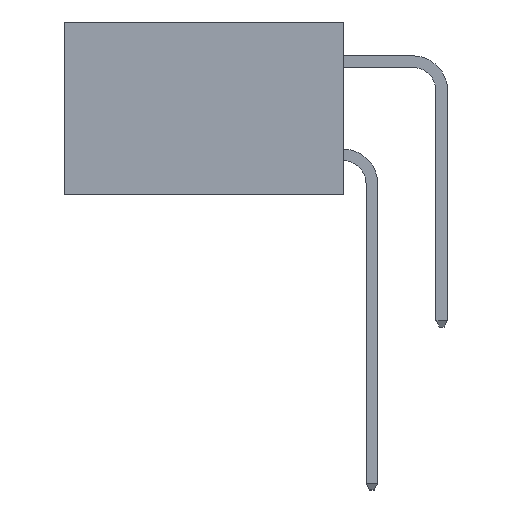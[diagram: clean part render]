
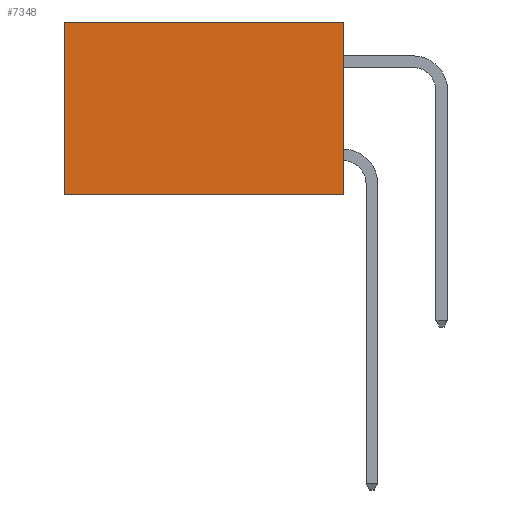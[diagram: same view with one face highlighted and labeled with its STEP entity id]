
A CAD part, left-side view. The second image highlights one B-rep face of the part: STEP entity #7348.
In plain terms, the highlighted planar face has unit normal (-1, 0, 0).
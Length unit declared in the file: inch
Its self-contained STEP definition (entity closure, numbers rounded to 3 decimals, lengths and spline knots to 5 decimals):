
#377 = VERTEX_POINT ( 'NONE', #873 ) ;
#873 = CARTESIAN_POINT ( 'NONE',  ( 0.2615, 0.6, -0.37 ) ) ;
#1054 = CARTESIAN_POINT ( 'NONE',  ( 0.2615, 0., -0.37 ) ) ;
#1093 = CARTESIAN_POINT ( 'NONE',  ( 0.2615, 0.6, -0.37 ) ) ;
#1723 = VERTEX_POINT ( 'NONE', #9330 ) ;
#3176 = VECTOR ( 'NONE', #5447, 39.37008 ) ;
#3414 = EDGE_CURVE ( 'NONE', #15702, #1723, #23495, .T. ) ;
#3593 = ORIENTED_EDGE ( 'NONE', *, *, #3872, .T. ) ;
#3872 = EDGE_CURVE ( 'NONE', #24324, #377, #17095, .T. ) ;
#5321 = VECTOR ( 'NONE', #11479, 39.37008 ) ;
#5447 = DIRECTION ( 'NONE',  ( 0., 1., 0. ) ) ;
#6010 = ORIENTED_EDGE ( 'NONE', *, *, #14614, .F. ) ;
#7329 = DIRECTION ( 'NONE',  ( 0., 0., -1. ) ) ;
#7348 = ADVANCED_FACE ( 'NONE', ( #12982 ), #21731, .F. ) ;
#7848 = CARTESIAN_POINT ( 'NONE',  ( 0.2615, 0., -0.37 ) ) ;
#9330 = CARTESIAN_POINT ( 'NONE',  ( 0.2615, 0., -0.37 ) ) ;
#9938 = DIRECTION ( 'NONE',  ( 0., 0., -1. ) ) ;
#11479 = DIRECTION ( 'NONE',  ( 0., 0., -1. ) ) ;
#11691 = CARTESIAN_POINT ( 'NONE',  ( 0.2615, 0., -0.37 ) ) ;
#12982 = FACE_OUTER_BOUND ( 'NONE', #26385, .T. ) ;
#14094 = CARTESIAN_POINT ( 'NONE',  ( 0.2615, 0.6, 0. ) ) ;
#14308 = LINE ( 'NONE', #11691, #3176 ) ;
#14614 = EDGE_CURVE ( 'NONE', #1723, #377, #14308, .T. ) ;
#14635 = CARTESIAN_POINT ( 'NONE',  ( 0.2615, 0., 0. ) ) ;
#15121 = LINE ( 'NONE', #14635, #24754 ) ;
#15158 = ORIENTED_EDGE ( 'NONE', *, *, #22772, .T. ) ;
#15702 = VERTEX_POINT ( 'NONE', #17273 ) ;
#16364 = AXIS2_PLACEMENT_3D ( 'NONE', #1054, #19769, #7329 ) ;
#17095 = LINE ( 'NONE', #1093, #5321 ) ;
#17273 = CARTESIAN_POINT ( 'NONE',  ( 0.2615, 0., 0. ) ) ;
#18965 = ORIENTED_EDGE ( 'NONE', *, *, #3414, .F. ) ;
#19769 = DIRECTION ( 'NONE',  ( 1., 0., 0. ) ) ;
#21731 = PLANE ( 'NONE',  #16364 ) ;
#22772 = EDGE_CURVE ( 'NONE', #15702, #24324, #15121, .T. ) ;
#22871 = VECTOR ( 'NONE', #9938, 39.37008 ) ;
#22884 = DIRECTION ( 'NONE',  ( 0., 1., 0. ) ) ;
#23495 = LINE ( 'NONE', #7848, #22871 ) ;
#24324 = VERTEX_POINT ( 'NONE', #14094 ) ;
#24754 = VECTOR ( 'NONE', #22884, 39.37008 ) ;
#26385 = EDGE_LOOP ( 'NONE', ( #3593, #6010, #18965, #15158 ) ) ;
